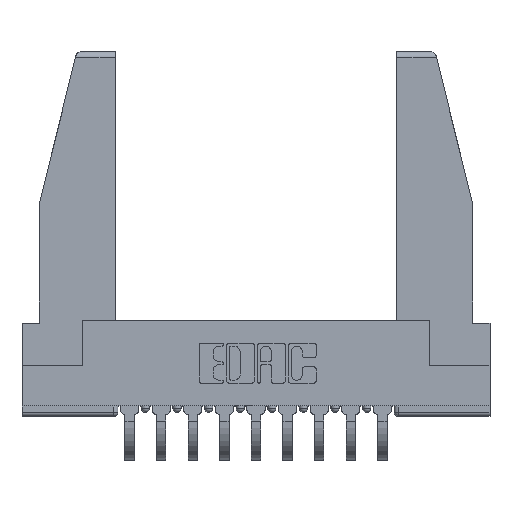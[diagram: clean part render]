
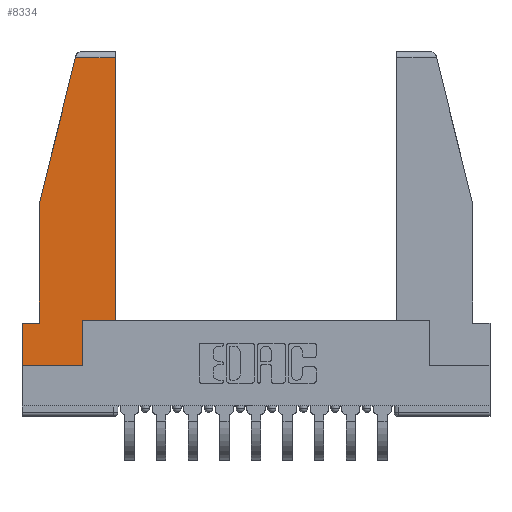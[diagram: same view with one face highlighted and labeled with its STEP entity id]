
A CAD part, top view. The second image highlights one B-rep face of the part: STEP entity #8334.
In plain terms, the highlighted planar face has unit normal (0, 0, 1).
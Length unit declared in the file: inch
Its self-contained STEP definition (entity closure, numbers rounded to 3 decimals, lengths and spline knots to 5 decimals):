
#172 = ORIENTED_EDGE ( 'NONE', *, *, #13168, .T. ) ;
#344 = ORIENTED_EDGE ( 'NONE', *, *, #10055, .T. ) ;
#362 = DIRECTION ( 'NONE',  ( -1., 0., 0. ) ) ;
#441 = DIRECTION ( 'NONE',  ( 1., 0., 0. ) ) ;
#668 = DIRECTION ( 'NONE',  ( 0., 1., 0. ) ) ;
#743 = CARTESIAN_POINT ( 'NONE',  ( 0., 0., 0. ) ) ;
#1638 = DIRECTION ( 'NONE',  ( -0.239, -0.971, 0. ) ) ;
#1976 = LINE ( 'NONE', #6688, #8451 ) ;
#2226 = VECTOR ( 'NONE', #668, 39.37008 ) ;
#2742 = LINE ( 'NONE', #7689, #10337 ) ;
#3280 = CARTESIAN_POINT ( 'NONE',  ( 0.297, 0., 0. ) ) ;
#3624 = VERTEX_POINT ( 'NONE', #3280 ) ;
#4050 = VECTOR ( 'NONE', #9286, 39.37008 ) ;
#4346 = CARTESIAN_POINT ( 'NONE',  ( 0.297, 0.223, 0. ) ) ;
#4721 = DIRECTION ( 'NONE',  ( 1., 0., 0. ) ) ;
#4765 = VECTOR ( 'NONE', #1638, 39.37008 ) ;
#4988 = VECTOR ( 'NONE', #10566, 39.37008 ) ;
#4998 = EDGE_LOOP ( 'NONE', ( #12751, #344, #9794, #172, #8212, #14343, #11665, #15113, #15798 ) ) ;
#5163 = CARTESIAN_POINT ( 'NONE',  ( 0., 0.21, 0. ) ) ;
#5280 = VERTEX_POINT ( 'NONE', #10328 ) ;
#5381 = LINE ( 'NONE', #7572, #4765 ) ;
#5482 = LINE ( 'NONE', #14105, #4988 ) ;
#6013 = DIRECTION ( 'NONE',  ( 0., 1., 0. ) ) ;
#6538 = CARTESIAN_POINT ( 'NONE',  ( 0., 0., 0. ) ) ;
#6688 = CARTESIAN_POINT ( 'NONE',  ( 0.086, 0.8, 0. ) ) ;
#6845 = CARTESIAN_POINT ( 'NONE',  ( 0.461, 0.223, 0. ) ) ;
#6991 = FACE_OUTER_BOUND ( 'NONE', #4998, .T. ) ;
#7228 = DIRECTION ( 'NONE',  ( 0., 0., 1. ) ) ;
#7572 = CARTESIAN_POINT ( 'NONE',  ( 0.271, 1.55, 0. ) ) ;
#7602 = DIRECTION ( 'NONE',  ( 0., -1., 0. ) ) ;
#7675 = LINE ( 'NONE', #5163, #12083 ) ;
#7689 = CARTESIAN_POINT ( 'NONE',  ( 0., 0.21, 0. ) ) ;
#8212 = ORIENTED_EDGE ( 'NONE', *, *, #15240, .T. ) ;
#8334 = ADVANCED_FACE ( 'NONE', ( #6991 ), #10697, .T. ) ;
#8451 = VECTOR ( 'NONE', #11600, 39.37008 ) ;
#9077 = EDGE_CURVE ( 'NONE', #10429, #14865, #2742, .T. ) ;
#9109 = CARTESIAN_POINT ( 'NONE',  ( 0., 0.21, 0. ) ) ;
#9126 = LINE ( 'NONE', #6538, #12956 ) ;
#9272 = CARTESIAN_POINT ( 'NONE',  ( 0.461, 1.52, 0. ) ) ;
#9286 = DIRECTION ( 'NONE',  ( 1., 0., 0. ) ) ;
#9359 = LINE ( 'NONE', #6845, #2226 ) ;
#9516 = EDGE_CURVE ( 'NONE', #14865, #3624, #9126, .T. ) ;
#9638 = VERTEX_POINT ( 'NONE', #14178 ) ;
#9794 = ORIENTED_EDGE ( 'NONE', *, *, #15697, .T. ) ;
#9865 = CARTESIAN_POINT ( 'NONE',  ( 0.086, 0.21, 0. ) ) ;
#10055 = EDGE_CURVE ( 'NONE', #15842, #14134, #5482, .T. ) ;
#10328 = CARTESIAN_POINT ( 'NONE',  ( 0.297, 0.223, 0. ) ) ;
#10337 = VECTOR ( 'NONE', #7602, 39.37008 ) ;
#10429 = VERTEX_POINT ( 'NONE', #9109 ) ;
#10488 = LINE ( 'NONE', #4346, #4050 ) ;
#10566 = DIRECTION ( 'NONE',  ( -1., 0., 0. ) ) ;
#10697 = PLANE ( 'NONE',  #13949 ) ;
#11004 = LINE ( 'NONE', #14311, #12513 ) ;
#11600 = DIRECTION ( 'NONE',  ( 0., -1., 0. ) ) ;
#11665 = ORIENTED_EDGE ( 'NONE', *, *, #9516, .T. ) ;
#12083 = VECTOR ( 'NONE', #362, 39.37008 ) ;
#12366 = EDGE_CURVE ( 'NONE', #3624, #5280, #11004, .T. ) ;
#12470 = VERTEX_POINT ( 'NONE', #13495 ) ;
#12513 = VECTOR ( 'NONE', #6013, 39.37008 ) ;
#12751 = ORIENTED_EDGE ( 'NONE', *, *, #13129, .T. ) ;
#12956 = VECTOR ( 'NONE', #441, 39.37008 ) ;
#13129 = EDGE_CURVE ( 'NONE', #12470, #15842, #9359, .T. ) ;
#13168 = EDGE_CURVE ( 'NONE', #9638, #15172, #1976, .T. ) ;
#13214 = CARTESIAN_POINT ( 'NONE',  ( 0.2636, 1.52, 0. ) ) ;
#13495 = CARTESIAN_POINT ( 'NONE',  ( 0.461, 0.223, 0. ) ) ;
#13949 = AXIS2_PLACEMENT_3D ( 'NONE', #743, #7228, #4721 ) ;
#14105 = CARTESIAN_POINT ( 'NONE',  ( 0., 1.52, 0. ) ) ;
#14128 = EDGE_CURVE ( 'NONE', #5280, #12470, #10488, .T. ) ;
#14134 = VERTEX_POINT ( 'NONE', #13214 ) ;
#14178 = CARTESIAN_POINT ( 'NONE',  ( 0.086, 0.8, 0. ) ) ;
#14311 = CARTESIAN_POINT ( 'NONE',  ( 0.297, 0., 0. ) ) ;
#14343 = ORIENTED_EDGE ( 'NONE', *, *, #9077, .T. ) ;
#14865 = VERTEX_POINT ( 'NONE', #14882 ) ;
#14882 = CARTESIAN_POINT ( 'NONE',  ( 0., 0., 0. ) ) ;
#15113 = ORIENTED_EDGE ( 'NONE', *, *, #12366, .T. ) ;
#15172 = VERTEX_POINT ( 'NONE', #9865 ) ;
#15240 = EDGE_CURVE ( 'NONE', #15172, #10429, #7675, .T. ) ;
#15697 = EDGE_CURVE ( 'NONE', #14134, #9638, #5381, .T. ) ;
#15798 = ORIENTED_EDGE ( 'NONE', *, *, #14128, .T. ) ;
#15842 = VERTEX_POINT ( 'NONE', #9272 ) ;
